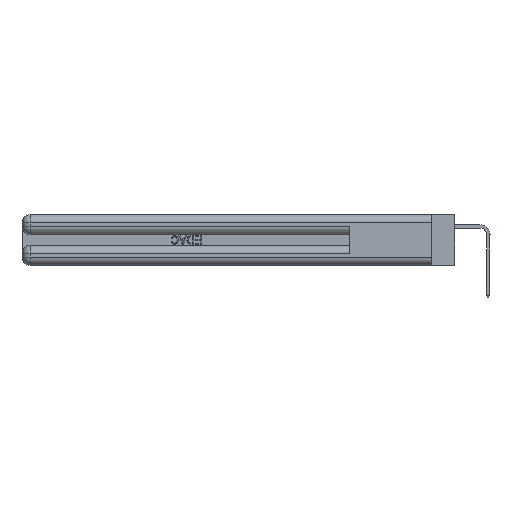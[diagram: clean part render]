
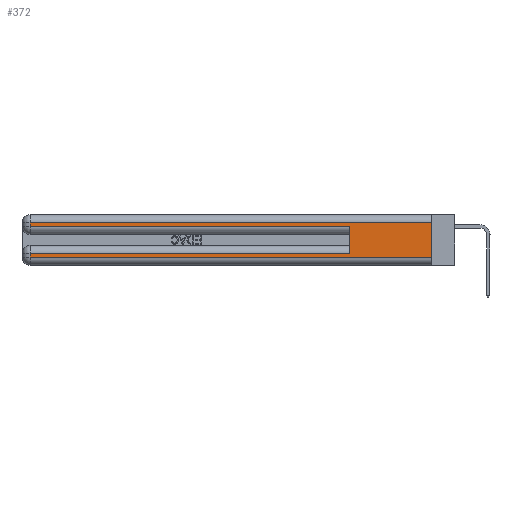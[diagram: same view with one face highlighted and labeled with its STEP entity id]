
A CAD part, left-side view. The second image highlights one B-rep face of the part: STEP entity #372.
In plain terms, the highlighted planar face has unit normal (-1, 0, 0).
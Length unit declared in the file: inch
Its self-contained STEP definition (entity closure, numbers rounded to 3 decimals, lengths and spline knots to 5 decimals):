
#372 = ADVANCED_FACE ( 'NONE', ( #29249 ), #14764, .F. ) ;
#727 = VECTOR ( 'NONE', #23677, 39.37008 ) ;
#1031 = CARTESIAN_POINT ( 'NONE',  ( 0., 2.94, 0.31 ) ) ;
#2981 = VERTEX_POINT ( 'NONE', #42223 ) ;
#3099 = CARTESIAN_POINT ( 'NONE',  ( 0., 0., 0.285 ) ) ;
#3651 = CARTESIAN_POINT ( 'NONE',  ( 0., 2.94, 0.285 ) ) ;
#3686 = LINE ( 'NONE', #20984, #20954 ) ;
#4190 = LINE ( 'NONE', #20739, #29456 ) ;
#4629 = VERTEX_POINT ( 'NONE', #1031 ) ;
#4990 = CARTESIAN_POINT ( 'NONE',  ( 0., 0., 0.31 ) ) ;
#6859 = DIRECTION ( 'NONE',  ( 0., 0., 1. ) ) ;
#7534 = VERTEX_POINT ( 'NONE', #44331 ) ;
#7874 = ORIENTED_EDGE ( 'NONE', *, *, #39019, .F. ) ;
#8422 = AXIS2_PLACEMENT_3D ( 'NONE', #11312, #28388, #18207 ) ;
#9505 = LINE ( 'NONE', #3099, #35658 ) ;
#9969 = DIRECTION ( 'NONE',  ( 0., -1., 0. ) ) ;
#10017 = LINE ( 'NONE', #30349, #727 ) ;
#10116 = EDGE_CURVE ( 'NONE', #35629, #2981, #9505, .T. ) ;
#10491 = CARTESIAN_POINT ( 'NONE',  ( 0., 0., 0.06 ) ) ;
#11312 = CARTESIAN_POINT ( 'NONE',  ( 0., 0., 0.37 ) ) ;
#12550 = VECTOR ( 'NONE', #20695, 39.37008 ) ;
#14208 = EDGE_CURVE ( 'NONE', #7534, #21507, #4190, .T. ) ;
#14269 = LINE ( 'NONE', #16390, #40343 ) ;
#14764 = PLANE ( 'NONE',  #8422 ) ;
#16175 = ORIENTED_EDGE ( 'NONE', *, *, #19994, .T. ) ;
#16336 = EDGE_CURVE ( 'NONE', #4629, #35629, #14269, .T. ) ;
#16390 = CARTESIAN_POINT ( 'NONE',  ( 0., 2.94, 0.37 ) ) ;
#17237 = CARTESIAN_POINT ( 'NONE',  ( 0., 0., 0.085 ) ) ;
#17335 = DIRECTION ( 'NONE',  ( 0., 0., -1. ) ) ;
#18207 = DIRECTION ( 'NONE',  ( 0., 0., -1. ) ) ;
#19994 = EDGE_CURVE ( 'NONE', #24416, #4629, #10017, .T. ) ;
#20695 = DIRECTION ( 'NONE',  ( 0., 1., 0. ) ) ;
#20739 = CARTESIAN_POINT ( 'NONE',  ( 0., 0., 0.06 ) ) ;
#20954 = VECTOR ( 'NONE', #24432, 39.37008 ) ;
#20984 = CARTESIAN_POINT ( 'NONE',  ( 0., 0., 0.37 ) ) ;
#21066 = CARTESIAN_POINT ( 'NONE',  ( 0., 2.94, 0.085 ) ) ;
#21489 = EDGE_CURVE ( 'NONE', #26170, #43541, #29688, .T. ) ;
#21507 = VERTEX_POINT ( 'NONE', #10491 ) ;
#22131 = EDGE_CURVE ( 'NONE', #43541, #7534, #32249, .T. ) ;
#23251 = VECTOR ( 'NONE', #17335, 39.37008 ) ;
#23677 = DIRECTION ( 'NONE',  ( 0., 1., 0. ) ) ;
#24035 = EDGE_LOOP ( 'NONE', ( #34215, #16175, #40210, #34403, #7874, #25388, #32096, #43435 ) ) ;
#24198 = DIRECTION ( 'NONE',  ( 0., -1., 0. ) ) ;
#24416 = VERTEX_POINT ( 'NONE', #4990 ) ;
#24432 = DIRECTION ( 'NONE',  ( 0., 0., -1. ) ) ;
#25155 = VECTOR ( 'NONE', #6859, 39.37008 ) ;
#25388 = ORIENTED_EDGE ( 'NONE', *, *, #21489, .T. ) ;
#26170 = VERTEX_POINT ( 'NONE', #32410 ) ;
#27440 = CARTESIAN_POINT ( 'NONE',  ( 0., 0.6, 0.145 ) ) ;
#28388 = DIRECTION ( 'NONE',  ( 1., 0., 0. ) ) ;
#29249 = FACE_OUTER_BOUND ( 'NONE', #24035, .T. ) ;
#29456 = VECTOR ( 'NONE', #24198, 39.37008 ) ;
#29688 = LINE ( 'NONE', #17237, #12550 ) ;
#30349 = CARTESIAN_POINT ( 'NONE',  ( 0., 0., 0.31 ) ) ;
#32096 = ORIENTED_EDGE ( 'NONE', *, *, #22131, .T. ) ;
#32249 = LINE ( 'NONE', #34294, #23251 ) ;
#32410 = CARTESIAN_POINT ( 'NONE',  ( 0., 0.6, 0.085 ) ) ;
#34215 = ORIENTED_EDGE ( 'NONE', *, *, #37577, .F. ) ;
#34294 = CARTESIAN_POINT ( 'NONE',  ( 0., 2.94, 0.37 ) ) ;
#34403 = ORIENTED_EDGE ( 'NONE', *, *, #10116, .T. ) ;
#35629 = VERTEX_POINT ( 'NONE', #3651 ) ;
#35658 = VECTOR ( 'NONE', #9969, 39.37008 ) ;
#36804 = DIRECTION ( 'NONE',  ( 0., 0., -1. ) ) ;
#37577 = EDGE_CURVE ( 'NONE', #24416, #21507, #3686, .T. ) ;
#39019 = EDGE_CURVE ( 'NONE', #26170, #2981, #42166, .T. ) ;
#40210 = ORIENTED_EDGE ( 'NONE', *, *, #16336, .T. ) ;
#40343 = VECTOR ( 'NONE', #36804, 39.37008 ) ;
#42166 = LINE ( 'NONE', #27440, #25155 ) ;
#42223 = CARTESIAN_POINT ( 'NONE',  ( 0., 0.6, 0.285 ) ) ;
#43435 = ORIENTED_EDGE ( 'NONE', *, *, #14208, .T. ) ;
#43541 = VERTEX_POINT ( 'NONE', #21066 ) ;
#44331 = CARTESIAN_POINT ( 'NONE',  ( 0., 2.94, 0.06 ) ) ;
